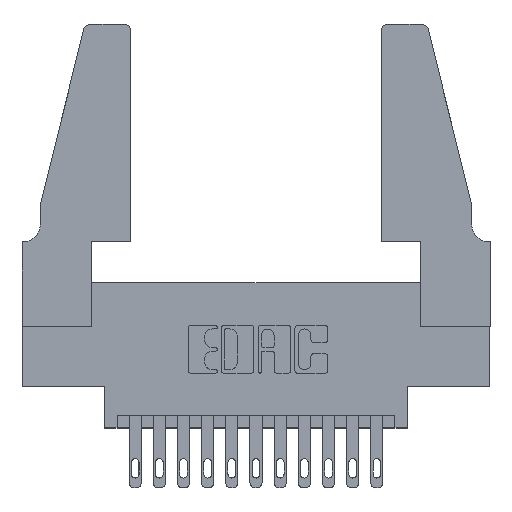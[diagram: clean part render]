
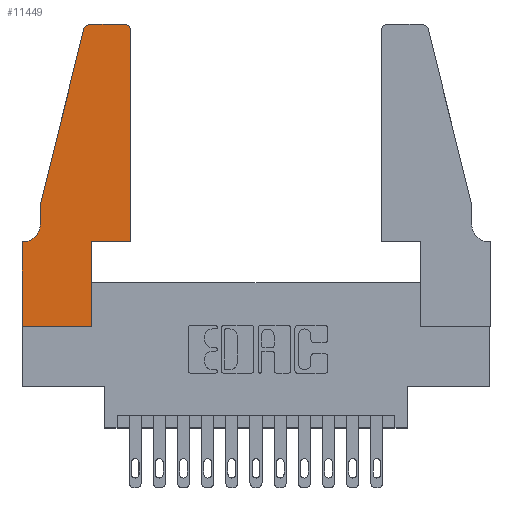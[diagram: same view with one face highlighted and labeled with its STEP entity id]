
A CAD part, top view. The second image highlights one B-rep face of the part: STEP entity #11449.
In plain terms, the highlighted planar face has unit normal (0, 0, 1).
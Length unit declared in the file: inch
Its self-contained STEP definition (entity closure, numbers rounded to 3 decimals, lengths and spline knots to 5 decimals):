
#23 = EDGE_CURVE ( 'NONE', #11634, #7910, #2119, .T. ) ;
#44 = EDGE_CURVE ( 'NONE', #10971, #6887, #4158, .T. ) ;
#292 = CARTESIAN_POINT ( 'NONE',  ( 0.284, 1.22, 0.37 ) ) ;
#299 = EDGE_CURVE ( 'NONE', #5135, #7365, #7395, .T. ) ;
#465 = DIRECTION ( 'NONE',  ( -1., 0., 0. ) ) ;
#472 = DIRECTION ( 'NONE',  ( 0., 1., 0. ) ) ;
#484 = CARTESIAN_POINT ( 'NONE',  ( 0.2865, 0., 0.37 ) ) ;
#606 = DIRECTION ( 'NONE',  ( 0., 0., 1. ) ) ;
#998 = DIRECTION ( 'NONE',  ( 1., 0., 0. ) ) ;
#1049 = VECTOR ( 'NONE', #6173, 39.37008 ) ;
#1157 = LINE ( 'NONE', #1579, #10035 ) ;
#1579 = CARTESIAN_POINT ( 'NONE',  ( 0.4505, 0.35, 0.37 ) ) ;
#1685 = CARTESIAN_POINT ( 'NONE',  ( 0.0055, 0.42, 0.37 ) ) ;
#1971 = CARTESIAN_POINT ( 'NONE',  ( 0., 0., 0.37 ) ) ;
#2119 = LINE ( 'NONE', #9619, #12073 ) ;
#2131 = CIRCLE ( 'NONE', #6942, 0.07 ) ;
#2258 = CARTESIAN_POINT ( 'NONE',  ( 0.284, 1.25, 0.37 ) ) ;
#2263 = ORIENTED_EDGE ( 'NONE', *, *, #4786, .T. ) ;
#2662 = AXIS2_PLACEMENT_3D ( 'NONE', #292, #8406, #4873 ) ;
#2743 = VERTEX_POINT ( 'NONE', #1971 ) ;
#2863 = LINE ( 'NONE', #11383, #9010 ) ;
#2938 = PLANE ( 'NONE',  #8584 ) ;
#2965 = ORIENTED_EDGE ( 'NONE', *, *, #10036, .T. ) ;
#3008 = ORIENTED_EDGE ( 'NONE', *, *, #4844, .T. ) ;
#3200 = CARTESIAN_POINT ( 'NONE',  ( 0.0755, 0.35, 0.37 ) ) ;
#3204 = CIRCLE ( 'NONE', #14784, 0.03 ) ;
#3320 = EDGE_CURVE ( 'NONE', #10595, #10971, #13498, .T. ) ;
#3609 = ORIENTED_EDGE ( 'NONE', *, *, #3320, .T. ) ;
#4123 = VECTOR ( 'NONE', #7976, 39.37008 ) ;
#4158 = LINE ( 'NONE', #8472, #10985 ) ;
#4786 = EDGE_CURVE ( 'NONE', #7910, #5429, #10909, .T. ) ;
#4844 = EDGE_CURVE ( 'NONE', #5429, #8251, #8415, .T. ) ;
#4873 = DIRECTION ( 'NONE',  ( 1., 0., 0. ) ) ;
#4880 = LINE ( 'NONE', #5485, #13901 ) ;
#5135 = VERTEX_POINT ( 'NONE', #5521 ) ;
#5287 = DIRECTION ( 'NONE',  ( 0., 0., -1. ) ) ;
#5429 = VERTEX_POINT ( 'NONE', #9622 ) ;
#5485 = CARTESIAN_POINT ( 'NONE',  ( 0., 0., 0.37 ) ) ;
#5521 = CARTESIAN_POINT ( 'NONE',  ( 0.0055, 0.35, 0.37 ) ) ;
#5709 = ORIENTED_EDGE ( 'NONE', *, *, #8836, .T. ) ;
#5727 = DIRECTION ( 'NONE',  ( -1., 0., 0. ) ) ;
#5785 = VERTEX_POINT ( 'NONE', #9198 ) ;
#5947 = DIRECTION ( 'NONE',  ( 1., 0., 0. ) ) ;
#6173 = DIRECTION ( 'NONE',  ( 0., -1., 0. ) ) ;
#6390 = ORIENTED_EDGE ( 'NONE', *, *, #9317, .T. ) ;
#6491 = CARTESIAN_POINT ( 'NONE',  ( 0., 0.35, 0.37 ) ) ;
#6544 = EDGE_LOOP ( 'NONE', ( #11268, #2263, #3008, #5709, #13050, #7785, #7055, #7762, #3609, #10942, #2965, #6390 ) ) ;
#6887 = VERTEX_POINT ( 'NONE', #9262 ) ;
#6942 = AXIS2_PLACEMENT_3D ( 'NONE', #1685, #5287, #5727 ) ;
#7055 = ORIENTED_EDGE ( 'NONE', *, *, #7842, .T. ) ;
#7124 = DIRECTION ( 'NONE',  ( 0., 0., 1. ) ) ;
#7365 = VERTEX_POINT ( 'NONE', #10059 ) ;
#7395 = LINE ( 'NONE', #3200, #12060 ) ;
#7586 = CARTESIAN_POINT ( 'NONE',  ( 0.2865, 0.35, 0.37 ) ) ;
#7701 = CARTESIAN_POINT ( 'NONE',  ( 0.4205, 1.25, 0.37 ) ) ;
#7762 = ORIENTED_EDGE ( 'NONE', *, *, #14134, .T. ) ;
#7785 = ORIENTED_EDGE ( 'NONE', *, *, #299, .T. ) ;
#7842 = EDGE_CURVE ( 'NONE', #7365, #2743, #4880, .T. ) ;
#7858 = VECTOR ( 'NONE', #14005, 39.37008 ) ;
#7910 = VERTEX_POINT ( 'NONE', #2258 ) ;
#7921 = CARTESIAN_POINT ( 'NONE',  ( 0.4505, 1.22, 0.37 ) ) ;
#7976 = DIRECTION ( 'NONE',  ( 0., 1., 0. ) ) ;
#8251 = VERTEX_POINT ( 'NONE', #8400 ) ;
#8400 = CARTESIAN_POINT ( 'NONE',  ( 0.0755, 0.5, 0.37 ) ) ;
#8406 = DIRECTION ( 'NONE',  ( 0., 0., 1. ) ) ;
#8415 = LINE ( 'NONE', #11658, #7858 ) ;
#8472 = CARTESIAN_POINT ( 'NONE',  ( 0.4505, 0.35, 0.37 ) ) ;
#8584 = AXIS2_PLACEMENT_3D ( 'NONE', #6491, #606, #13345 ) ;
#8836 = EDGE_CURVE ( 'NONE', #8251, #5785, #9015, .T. ) ;
#9010 = VECTOR ( 'NONE', #998, 39.37008 ) ;
#9015 = LINE ( 'NONE', #14151, #1049 ) ;
#9198 = CARTESIAN_POINT ( 'NONE',  ( 0.0755, 0.42, 0.37 ) ) ;
#9262 = CARTESIAN_POINT ( 'NONE',  ( 0.4505, 0.35, 0.37 ) ) ;
#9317 = EDGE_CURVE ( 'NONE', #14216, #11634, #3204, .T. ) ;
#9619 = CARTESIAN_POINT ( 'NONE',  ( 0.2605, 1.25, 0.37 ) ) ;
#9622 = CARTESIAN_POINT ( 'NONE',  ( 0.25487, 1.22718, 0.37 ) ) ;
#10035 = VECTOR ( 'NONE', #472, 39.37008 ) ;
#10036 = EDGE_CURVE ( 'NONE', #6887, #14216, #1157, .T. ) ;
#10059 = CARTESIAN_POINT ( 'NONE',  ( 0., 0.35, 0.37 ) ) ;
#10526 = CARTESIAN_POINT ( 'NONE',  ( 0.4205, 1.22, 0.37 ) ) ;
#10595 = VERTEX_POINT ( 'NONE', #484 ) ;
#10909 = CIRCLE ( 'NONE', #2662, 0.03 ) ;
#10942 = ORIENTED_EDGE ( 'NONE', *, *, #44, .T. ) ;
#10971 = VERTEX_POINT ( 'NONE', #14140 ) ;
#10985 = VECTOR ( 'NONE', #14296, 39.37008 ) ;
#11056 = FACE_OUTER_BOUND ( 'NONE', #6544, .T. ) ;
#11199 = DIRECTION ( 'NONE',  ( -1., 0., 0. ) ) ;
#11268 = ORIENTED_EDGE ( 'NONE', *, *, #23, .T. ) ;
#11292 = DIRECTION ( 'NONE',  ( 0., -1., 0. ) ) ;
#11383 = CARTESIAN_POINT ( 'NONE',  ( 0., 0., 0.37 ) ) ;
#11449 = ADVANCED_FACE ( 'NONE', ( #11056 ), #2938, .T. ) ;
#11634 = VERTEX_POINT ( 'NONE', #7701 ) ;
#11658 = CARTESIAN_POINT ( 'NONE',  ( 0.0755, 0.5, 0.37 ) ) ;
#12060 = VECTOR ( 'NONE', #11199, 39.37008 ) ;
#12073 = VECTOR ( 'NONE', #465, 39.37008 ) ;
#12991 = EDGE_CURVE ( 'NONE', #5785, #5135, #2131, .T. ) ;
#13050 = ORIENTED_EDGE ( 'NONE', *, *, #12991, .T. ) ;
#13345 = DIRECTION ( 'NONE',  ( 1., 0., 0. ) ) ;
#13498 = LINE ( 'NONE', #7586, #4123 ) ;
#13901 = VECTOR ( 'NONE', #11292, 39.37008 ) ;
#14005 = DIRECTION ( 'NONE',  ( -0.239, -0.971, 0. ) ) ;
#14134 = EDGE_CURVE ( 'NONE', #2743, #10595, #2863, .T. ) ;
#14140 = CARTESIAN_POINT ( 'NONE',  ( 0.2865, 0.35, 0.37 ) ) ;
#14151 = CARTESIAN_POINT ( 'NONE',  ( 0.0755, 0.5, 0.37 ) ) ;
#14216 = VERTEX_POINT ( 'NONE', #7921 ) ;
#14296 = DIRECTION ( 'NONE',  ( 1., 0., 0. ) ) ;
#14784 = AXIS2_PLACEMENT_3D ( 'NONE', #10526, #7124, #5947 ) ;
